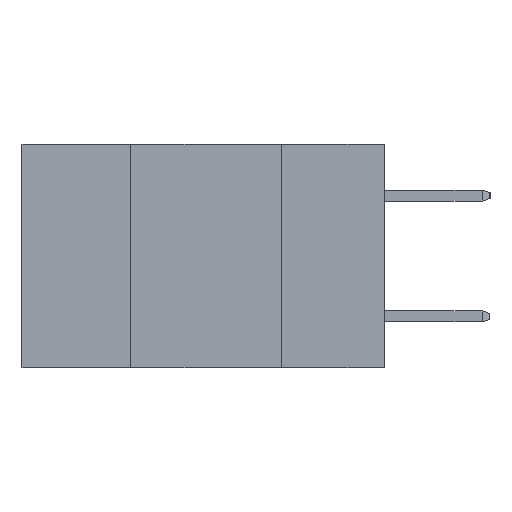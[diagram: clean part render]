
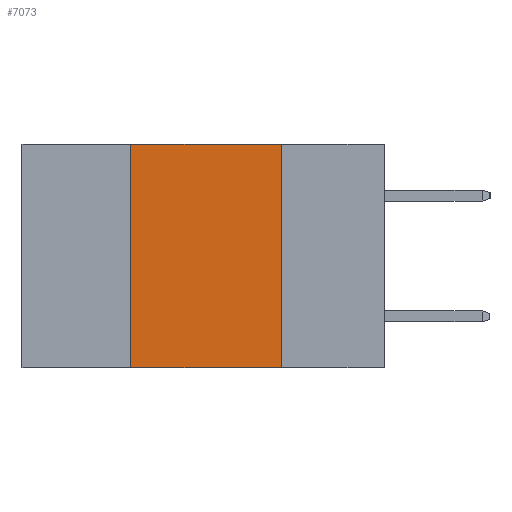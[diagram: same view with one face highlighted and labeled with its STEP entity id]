
A CAD part, left-side view. The second image highlights one B-rep face of the part: STEP entity #7073.
In plain terms, the highlighted planar face has unit normal (-1, 0, 0).
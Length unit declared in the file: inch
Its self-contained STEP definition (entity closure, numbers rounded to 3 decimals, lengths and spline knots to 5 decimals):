
#193 = DIRECTION ( 'NONE',  ( 0., 0., -1. ) ) ;
#534 = CARTESIAN_POINT ( 'NONE',  ( 0., 0.6, -0.37 ) ) ;
#808 = VERTEX_POINT ( 'NONE', #10807 ) ;
#1032 = ORIENTED_EDGE ( 'NONE', *, *, #11060, .F. ) ;
#1470 = LINE ( 'NONE', #10457, #12035 ) ;
#1516 = AXIS2_PLACEMENT_3D ( 'NONE', #10129, #6882, #8960 ) ;
#2689 = ORIENTED_EDGE ( 'NONE', *, *, #10373, .T. ) ;
#3177 = EDGE_CURVE ( 'NONE', #808, #3900, #8976, .T. ) ;
#3348 = ORIENTED_EDGE ( 'NONE', *, *, #3177, .F. ) ;
#3457 = VERTEX_POINT ( 'NONE', #12482 ) ;
#3714 = CARTESIAN_POINT ( 'NONE',  ( 0., 0.17, 0. ) ) ;
#3900 = VERTEX_POINT ( 'NONE', #3714 ) ;
#4064 = CARTESIAN_POINT ( 'NONE',  ( 0., 0.42, -0.37 ) ) ;
#4212 = CARTESIAN_POINT ( 'NONE',  ( 0., 0.42, 0. ) ) ;
#4311 = VERTEX_POINT ( 'NONE', #4064 ) ;
#4476 = DIRECTION ( 'NONE',  ( 0., -1., 0. ) ) ;
#4480 = ORIENTED_EDGE ( 'NONE', *, *, #11716, .F. ) ;
#4714 = EDGE_LOOP ( 'NONE', ( #4480, #3348, #1032, #2689 ) ) ;
#6882 = DIRECTION ( 'NONE',  ( 1., 0., 0. ) ) ;
#6994 = PLANE ( 'NONE',  #1516 ) ;
#7073 = ADVANCED_FACE ( 'NONE', ( #11410 ), #6994, .F. ) ;
#7192 = LINE ( 'NONE', #4212, #9853 ) ;
#7806 = DIRECTION ( 'NONE',  ( 0., -1., 0. ) ) ;
#7985 = LINE ( 'NONE', #534, #10663 ) ;
#8960 = DIRECTION ( 'NONE',  ( 0., 0., -1. ) ) ;
#8976 = LINE ( 'NONE', #12064, #11348 ) ;
#9853 = VECTOR ( 'NONE', #10290, 39.37008 ) ;
#10129 = CARTESIAN_POINT ( 'NONE',  ( 0., 0.6, 0. ) ) ;
#10290 = DIRECTION ( 'NONE',  ( 0., 0., 1. ) ) ;
#10373 = EDGE_CURVE ( 'NONE', #4311, #3457, #7985, .T. ) ;
#10457 = CARTESIAN_POINT ( 'NONE',  ( 0., 0.17, 0. ) ) ;
#10663 = VECTOR ( 'NONE', #7806, 39.37008 ) ;
#10807 = CARTESIAN_POINT ( 'NONE',  ( 0., 0.42, 0. ) ) ;
#11060 = EDGE_CURVE ( 'NONE', #4311, #808, #7192, .T. ) ;
#11348 = VECTOR ( 'NONE', #4476, 39.37008 ) ;
#11410 = FACE_OUTER_BOUND ( 'NONE', #4714, .T. ) ;
#11716 = EDGE_CURVE ( 'NONE', #3900, #3457, #1470, .T. ) ;
#12035 = VECTOR ( 'NONE', #193, 39.37008 ) ;
#12064 = CARTESIAN_POINT ( 'NONE',  ( 0., 0.6, 0. ) ) ;
#12482 = CARTESIAN_POINT ( 'NONE',  ( 0., 0.17, -0.37 ) ) ;
